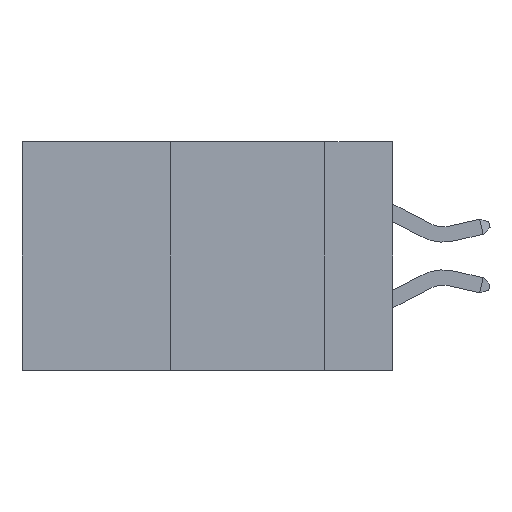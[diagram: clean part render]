
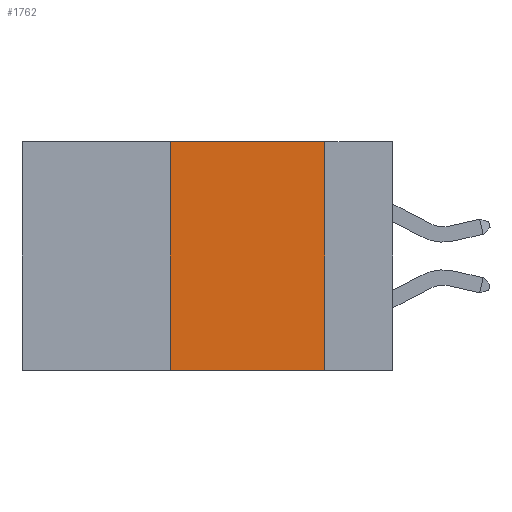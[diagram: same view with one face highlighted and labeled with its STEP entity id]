
A CAD part, left-side view. The second image highlights one B-rep face of the part: STEP entity #1762.
In plain terms, the highlighted planar face has unit normal (-1, 0, 0).
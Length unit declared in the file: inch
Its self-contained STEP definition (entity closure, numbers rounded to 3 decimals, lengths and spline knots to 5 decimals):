
#52 = CARTESIAN_POINT ( 'NONE',  ( 0., 0.11, 0. ) ) ;
#128 = LINE ( 'NONE', #13122, #13709 ) ;
#147 = EDGE_CURVE ( 'NONE', #5099, #11461, #12325, .T. ) ;
#1206 = EDGE_CURVE ( 'NONE', #5099, #4985, #3517, .T. ) ;
#1762 = ADVANCED_FACE ( 'NONE', ( #4524 ), #4821, .F. ) ;
#2723 = EDGE_CURVE ( 'NONE', #6738, #11461, #128, .T. ) ;
#2733 = DIRECTION ( 'NONE',  ( 0., -1., 0. ) ) ;
#3517 = LINE ( 'NONE', #9998, #6626 ) ;
#3751 = DIRECTION ( 'NONE',  ( 0., 0., 1. ) ) ;
#4093 = LINE ( 'NONE', #14798, #7612 ) ;
#4524 = FACE_OUTER_BOUND ( 'NONE', #12580, .T. ) ;
#4821 = PLANE ( 'NONE',  #10035 ) ;
#4985 = VERTEX_POINT ( 'NONE', #16008 ) ;
#5099 = VERTEX_POINT ( 'NONE', #12339 ) ;
#5296 = DIRECTION ( 'NONE',  ( 0., 0., -1. ) ) ;
#5445 = DIRECTION ( 'NONE',  ( 1., 0., 0. ) ) ;
#5506 = CARTESIAN_POINT ( 'NONE',  ( 0., 0.6, -0.37 ) ) ;
#5855 = CARTESIAN_POINT ( 'NONE',  ( 0., 0.6, 0. ) ) ;
#6626 = VECTOR ( 'NONE', #3751, 39.37008 ) ;
#6738 = VERTEX_POINT ( 'NONE', #52 ) ;
#7612 = VECTOR ( 'NONE', #2733, 39.37008 ) ;
#8822 = DIRECTION ( 'NONE',  ( 0., -1., 0. ) ) ;
#9998 = CARTESIAN_POINT ( 'NONE',  ( 0., 0.36, 0. ) ) ;
#10035 = AXIS2_PLACEMENT_3D ( 'NONE', #5855, #5445, #11063 ) ;
#11063 = DIRECTION ( 'NONE',  ( 0., 0., -1. ) ) ;
#11461 = VERTEX_POINT ( 'NONE', #12568 ) ;
#11877 = ORIENTED_EDGE ( 'NONE', *, *, #2723, .F. ) ;
#12325 = LINE ( 'NONE', #5506, #15804 ) ;
#12339 = CARTESIAN_POINT ( 'NONE',  ( 0., 0.36, -0.37 ) ) ;
#12568 = CARTESIAN_POINT ( 'NONE',  ( 0., 0.11, -0.37 ) ) ;
#12580 = EDGE_LOOP ( 'NONE', ( #11877, #14296, #14788, #15633 ) ) ;
#13122 = CARTESIAN_POINT ( 'NONE',  ( 0., 0.11, 0. ) ) ;
#13709 = VECTOR ( 'NONE', #5296, 39.37008 ) ;
#13819 = EDGE_CURVE ( 'NONE', #4985, #6738, #4093, .T. ) ;
#14296 = ORIENTED_EDGE ( 'NONE', *, *, #13819, .F. ) ;
#14788 = ORIENTED_EDGE ( 'NONE', *, *, #1206, .F. ) ;
#14798 = CARTESIAN_POINT ( 'NONE',  ( 0., 0.6, 0. ) ) ;
#15633 = ORIENTED_EDGE ( 'NONE', *, *, #147, .T. ) ;
#15804 = VECTOR ( 'NONE', #8822, 39.37008 ) ;
#16008 = CARTESIAN_POINT ( 'NONE',  ( 0., 0.36, 0. ) ) ;
